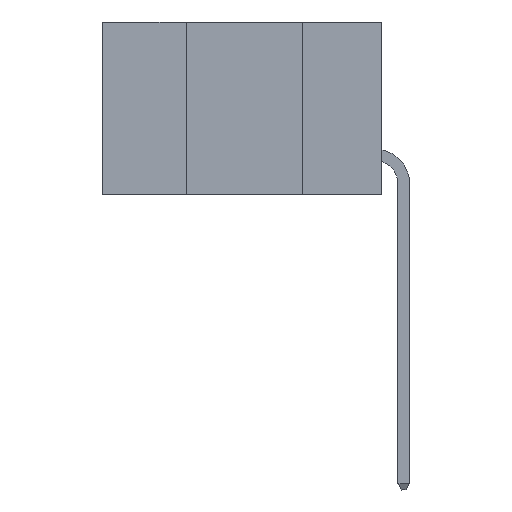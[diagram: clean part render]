
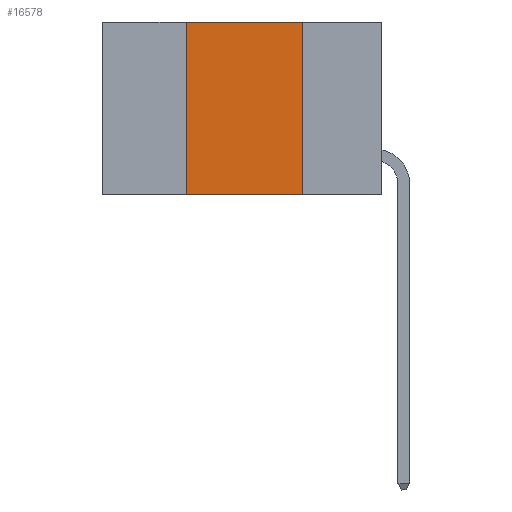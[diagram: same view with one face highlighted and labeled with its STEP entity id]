
A CAD part, left-side view. The second image highlights one B-rep face of the part: STEP entity #16578.
In plain terms, the highlighted planar face has unit normal (-1, 0, 0).
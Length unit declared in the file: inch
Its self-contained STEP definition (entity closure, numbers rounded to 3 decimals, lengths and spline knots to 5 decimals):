
#59 = LINE ( 'NONE', #17313, #16904 ) ;
#801 = DIRECTION ( 'NONE',  ( 0., -1., 0. ) ) ;
#2576 = CARTESIAN_POINT ( 'NONE',  ( 0., 0.6, 0. ) ) ;
#2657 = DIRECTION ( 'NONE',  ( 1., 0., 0. ) ) ;
#2733 = VERTEX_POINT ( 'NONE', #18129 ) ;
#2807 = EDGE_CURVE ( 'NONE', #12766, #2733, #16708, .T. ) ;
#3759 = EDGE_CURVE ( 'NONE', #2733, #4837, #59, .T. ) ;
#4799 = DIRECTION ( 'NONE',  ( 0., -1., 0. ) ) ;
#4837 = VERTEX_POINT ( 'NONE', #17367 ) ;
#5295 = VECTOR ( 'NONE', #801, 39.37008 ) ;
#5804 = FACE_OUTER_BOUND ( 'NONE', #7370, .T. ) ;
#5838 = CARTESIAN_POINT ( 'NONE',  ( 0., 0.42, 0. ) ) ;
#6278 = CARTESIAN_POINT ( 'NONE',  ( 0., 0.17, -0.37 ) ) ;
#6299 = ORIENTED_EDGE ( 'NONE', *, *, #3759, .F. ) ;
#6528 = AXIS2_PLACEMENT_3D ( 'NONE', #2576, #2657, #14112 ) ;
#6814 = EDGE_CURVE ( 'NONE', #12766, #7288, #14414, .T. ) ;
#7020 = ORIENTED_EDGE ( 'NONE', *, *, #6814, .T. ) ;
#7288 = VERTEX_POINT ( 'NONE', #6278 ) ;
#7370 = EDGE_LOOP ( 'NONE', ( #16741, #6299, #7596, #7020 ) ) ;
#7596 = ORIENTED_EDGE ( 'NONE', *, *, #2807, .F. ) ;
#8265 = EDGE_CURVE ( 'NONE', #4837, #7288, #18335, .T. ) ;
#8316 = VECTOR ( 'NONE', #8431, 39.37008 ) ;
#8431 = DIRECTION ( 'NONE',  ( 0., 0., 1. ) ) ;
#10135 = VECTOR ( 'NONE', #14801, 39.37008 ) ;
#10929 = PLANE ( 'NONE',  #6528 ) ;
#12766 = VERTEX_POINT ( 'NONE', #13047 ) ;
#13047 = CARTESIAN_POINT ( 'NONE',  ( 0., 0.42, -0.37 ) ) ;
#13252 = CARTESIAN_POINT ( 'NONE',  ( 0., 0.17, 0. ) ) ;
#14112 = DIRECTION ( 'NONE',  ( 0., 0., -1. ) ) ;
#14414 = LINE ( 'NONE', #14641, #5295 ) ;
#14641 = CARTESIAN_POINT ( 'NONE',  ( 0., 0.6, -0.37 ) ) ;
#14801 = DIRECTION ( 'NONE',  ( 0., 0., -1. ) ) ;
#16578 = ADVANCED_FACE ( 'NONE', ( #5804 ), #10929, .F. ) ;
#16708 = LINE ( 'NONE', #5838, #8316 ) ;
#16741 = ORIENTED_EDGE ( 'NONE', *, *, #8265, .F. ) ;
#16904 = VECTOR ( 'NONE', #4799, 39.37008 ) ;
#17313 = CARTESIAN_POINT ( 'NONE',  ( 0., 0.6, 0. ) ) ;
#17367 = CARTESIAN_POINT ( 'NONE',  ( 0., 0.17, 0. ) ) ;
#18129 = CARTESIAN_POINT ( 'NONE',  ( 0., 0.42, 0. ) ) ;
#18335 = LINE ( 'NONE', #13252, #10135 ) ;
